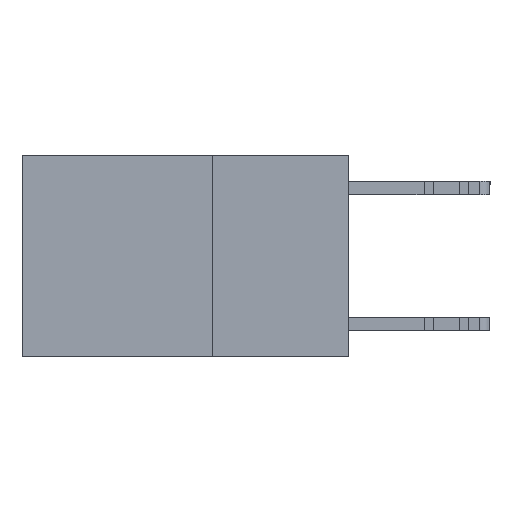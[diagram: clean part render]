
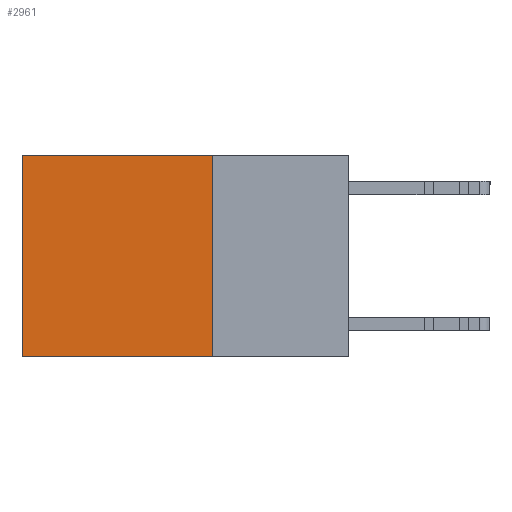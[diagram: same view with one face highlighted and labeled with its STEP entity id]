
A CAD part, left-side view. The second image highlights one B-rep face of the part: STEP entity #2961.
In plain terms, the highlighted planar face has unit normal (-1, 0, 0).
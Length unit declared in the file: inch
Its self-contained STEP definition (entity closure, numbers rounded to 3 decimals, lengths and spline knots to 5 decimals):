
#1944 = LINE ( 'NONE', #4445, #23078 ) ;
#2295 = EDGE_CURVE ( 'NONE', #28679, #24561, #1944, .T. ) ;
#2961 = ADVANCED_FACE ( 'NONE', ( #19040 ), #12449, .F. ) ;
#3595 = LINE ( 'NONE', #17200, #7764 ) ;
#3793 = LINE ( 'NONE', #19028, #26573 ) ;
#4445 = CARTESIAN_POINT ( 'NONE',  ( 0.2625, 0.25, 0. ) ) ;
#4674 = CARTESIAN_POINT ( 'NONE',  ( 0.2625, 0.6, 0. ) ) ;
#4724 = ORIENTED_EDGE ( 'NONE', *, *, #27302, .F. ) ;
#7086 = ORIENTED_EDGE ( 'NONE', *, *, #18967, .T. ) ;
#7756 = CARTESIAN_POINT ( 'NONE',  ( 0.2625, 0.25, 0. ) ) ;
#7764 = VECTOR ( 'NONE', #7975, 39.37008 ) ;
#7975 = DIRECTION ( 'NONE',  ( 0., 0., -1. ) ) ;
#9788 = VERTEX_POINT ( 'NONE', #10461 ) ;
#9803 = LINE ( 'NONE', #18762, #26889 ) ;
#9852 = EDGE_LOOP ( 'NONE', ( #7086, #21058, #4724, #18724 ) ) ;
#10461 = CARTESIAN_POINT ( 'NONE',  ( 0.2625, 0.6, -0.37 ) ) ;
#10590 = DIRECTION ( 'NONE',  ( 0., 1., 0. ) ) ;
#11952 = CARTESIAN_POINT ( 'NONE',  ( 0.2625, 0.25, -0.37 ) ) ;
#12163 = DIRECTION ( 'NONE',  ( 0., 0., -1. ) ) ;
#12449 = PLANE ( 'NONE',  #14289 ) ;
#14105 = VERTEX_POINT ( 'NONE', #11952 ) ;
#14289 = AXIS2_PLACEMENT_3D ( 'NONE', #7756, #16268, #12163 ) ;
#16268 = DIRECTION ( 'NONE',  ( 1., 0., 0. ) ) ;
#16565 = DIRECTION ( 'NONE',  ( 0., 1., 0. ) ) ;
#17113 = DIRECTION ( 'NONE',  ( 0., 0., -1. ) ) ;
#17200 = CARTESIAN_POINT ( 'NONE',  ( 0.2625, 0.6, 0. ) ) ;
#17980 = EDGE_CURVE ( 'NONE', #14105, #9788, #9803, .T. ) ;
#18724 = ORIENTED_EDGE ( 'NONE', *, *, #2295, .T. ) ;
#18762 = CARTESIAN_POINT ( 'NONE',  ( 0.2625, 0.25, -0.37 ) ) ;
#18967 = EDGE_CURVE ( 'NONE', #24561, #9788, #3595, .T. ) ;
#19028 = CARTESIAN_POINT ( 'NONE',  ( 0.2625, 0.25, 0. ) ) ;
#19040 = FACE_OUTER_BOUND ( 'NONE', #9852, .T. ) ;
#21058 = ORIENTED_EDGE ( 'NONE', *, *, #17980, .F. ) ;
#23078 = VECTOR ( 'NONE', #10590, 39.37008 ) ;
#24561 = VERTEX_POINT ( 'NONE', #4674 ) ;
#25762 = CARTESIAN_POINT ( 'NONE',  ( 0.2625, 0.25, 0. ) ) ;
#26573 = VECTOR ( 'NONE', #17113, 39.37008 ) ;
#26889 = VECTOR ( 'NONE', #16565, 39.37008 ) ;
#27302 = EDGE_CURVE ( 'NONE', #28679, #14105, #3793, .T. ) ;
#28679 = VERTEX_POINT ( 'NONE', #25762 ) ;
